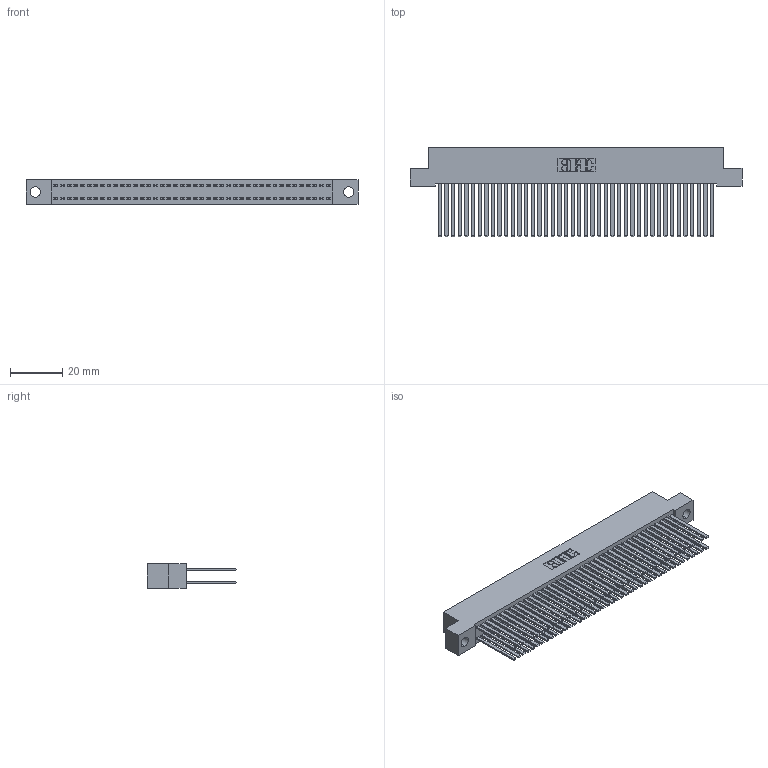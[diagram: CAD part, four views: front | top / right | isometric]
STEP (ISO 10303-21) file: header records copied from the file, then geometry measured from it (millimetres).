
FILE_DESCRIPTION (( 'STEP AP203' ), '1' );
FILE_NAME ('342-084-544-204.STEP', '2019-10-04T12:44:35', ( '' ), ( '' ), 'SwSTEP 2.0', 'SolidWorks 2016', '' );
FILE_SCHEMA (( 'CONFIG_CONTROL_DESIGN' ));
Length unit declared in the file: inch
Products named in the file (3): 342-084-544-204; 342 Part_.156 TH; 345-292-001_345-293-144
Assembly tree (85 placements, depth 2):
  342-084-544-204
    342 Part_.156 TH
    345-292-001_345-293-144  x84
Bounding box: 127 x 34.3 x 9.4 mm (x, y, z)
Volume: 12501.4 mm3; surface area: 23434.4 mm2
Topology: 85 solids, 85 shells, 3974 faces, 11807 edges, 7758 vertices
Faces by surface type: plane 2754, cylinder 1220
Entity records: 26707 total; most frequent: CARTESIAN_POINT 4422, ORIENTED_EDGE 4358, DIRECTION 3775, EDGE_CURVE 2179, LINE 2055, VECTOR 2055, VERTEX_POINT 1450, AXIS2_PLACEMENT_3D 860
